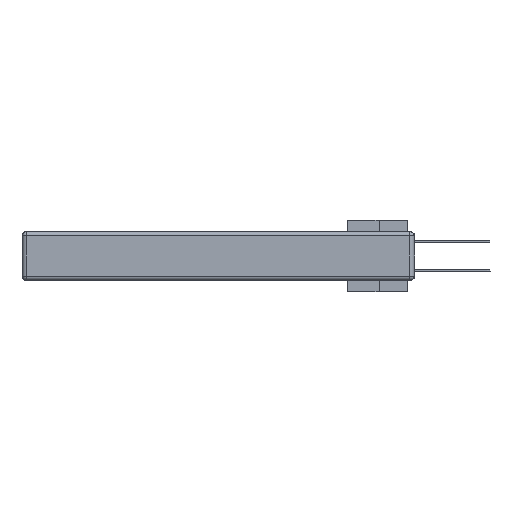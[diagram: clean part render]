
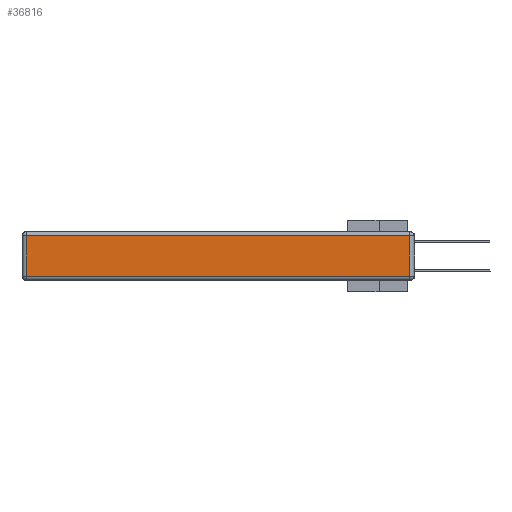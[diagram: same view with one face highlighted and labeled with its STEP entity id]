
A CAD part, left-side view. The second image highlights one B-rep face of the part: STEP entity #36816.
In plain terms, the highlighted planar face has unit normal (-1, 0, 0).
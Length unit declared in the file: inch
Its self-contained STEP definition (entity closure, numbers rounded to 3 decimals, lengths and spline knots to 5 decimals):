
#1022 = LINE ( 'NONE', #36564, #23807 ) ;
#2020 = CARTESIAN_POINT ( 'NONE',  ( 0., 0.03, -0.03 ) ) ;
#3009 = ORIENTED_EDGE ( 'NONE', *, *, #19682, .T. ) ;
#5698 = ORIENTED_EDGE ( 'NONE', *, *, #15933, .T. ) ;
#5718 = DIRECTION ( 'NONE',  ( 0., 1., 0. ) ) ;
#6809 = LINE ( 'NONE', #30831, #34880 ) ;
#9939 = DIRECTION ( 'NONE',  ( -1., 0., 0. ) ) ;
#10390 = CARTESIAN_POINT ( 'NONE',  ( 0., 2.72, -0.343 ) ) ;
#10641 = EDGE_LOOP ( 'NONE', ( #26916, #5698, #3009, #26051 ) ) ;
#11086 = AXIS2_PLACEMENT_3D ( 'NONE', #37269, #9939, #24993 ) ;
#11581 = LINE ( 'NONE', #14116, #16969 ) ;
#12539 = LINE ( 'NONE', #10390, #36089 ) ;
#13796 = EDGE_CURVE ( 'NONE', #36298, #33888, #12539, .T. ) ;
#14116 = CARTESIAN_POINT ( 'NONE',  ( 0., 2.75, -0.03 ) ) ;
#15403 = DIRECTION ( 'NONE',  ( 0., 0., 1. ) ) ;
#15933 = EDGE_CURVE ( 'NONE', #16996, #26386, #6809, .T. ) ;
#16183 = FACE_OUTER_BOUND ( 'NONE', #10641, .T. ) ;
#16656 = CARTESIAN_POINT ( 'NONE',  ( 0., 0.03, -0.313 ) ) ;
#16969 = VECTOR ( 'NONE', #5718, 39.37008 ) ;
#16996 = VERTEX_POINT ( 'NONE', #16656 ) ;
#18407 = CARTESIAN_POINT ( 'NONE',  ( 0., 2.72, -0.03 ) ) ;
#19682 = EDGE_CURVE ( 'NONE', #26386, #36298, #11581, .T. ) ;
#21559 = DIRECTION ( 'NONE',  ( 0., -1., 0. ) ) ;
#23807 = VECTOR ( 'NONE', #21559, 39.37008 ) ;
#24993 = DIRECTION ( 'NONE',  ( 0., 0., 1. ) ) ;
#26051 = ORIENTED_EDGE ( 'NONE', *, *, #13796, .T. ) ;
#26386 = VERTEX_POINT ( 'NONE', #2020 ) ;
#26916 = ORIENTED_EDGE ( 'NONE', *, *, #28014, .T. ) ;
#28014 = EDGE_CURVE ( 'NONE', #33888, #16996, #1022, .T. ) ;
#30831 = CARTESIAN_POINT ( 'NONE',  ( 0., 0.03, -0.343 ) ) ;
#31234 = PLANE ( 'NONE',  #11086 ) ;
#33888 = VERTEX_POINT ( 'NONE', #38201 ) ;
#34880 = VECTOR ( 'NONE', #15403, 39.37008 ) ;
#36089 = VECTOR ( 'NONE', #36573, 39.37008 ) ;
#36298 = VERTEX_POINT ( 'NONE', #18407 ) ;
#36564 = CARTESIAN_POINT ( 'NONE',  ( 0., 0., -0.313 ) ) ;
#36573 = DIRECTION ( 'NONE',  ( 0., 0., -1. ) ) ;
#36816 = ADVANCED_FACE ( 'NONE', ( #16183 ), #31234, .T. ) ;
#37269 = CARTESIAN_POINT ( 'NONE',  ( 0., 0., -0.343 ) ) ;
#38201 = CARTESIAN_POINT ( 'NONE',  ( 0., 2.72, -0.313 ) ) ;
